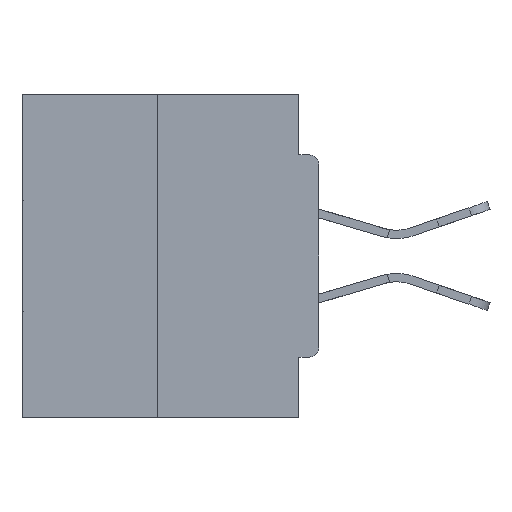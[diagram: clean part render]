
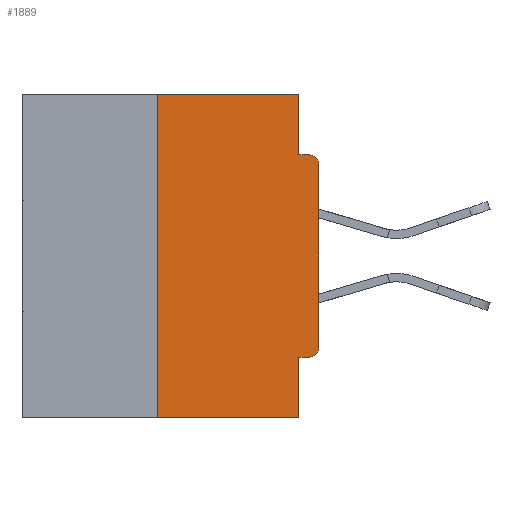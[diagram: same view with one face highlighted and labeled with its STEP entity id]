
A CAD part, left-side view. The second image highlights one B-rep face of the part: STEP entity #1889.
In plain terms, the highlighted planar face has unit normal (-1, 0, 0).
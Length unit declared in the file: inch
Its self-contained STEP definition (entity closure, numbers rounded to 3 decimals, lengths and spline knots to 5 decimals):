
#414 = CARTESIAN_POINT ( 'NONE',  ( 0., 0.015, -0.1085 ) ) ;
#616 = CARTESIAN_POINT ( 'NONE',  ( 0., 0., 0. ) ) ;
#1851 = VERTEX_POINT ( 'NONE', #23936 ) ;
#1889 = ADVANCED_FACE ( 'NONE', ( #33391 ), #14677, .F. ) ;
#1933 = CARTESIAN_POINT ( 'NONE',  ( 0., 0., -0.3915 ) ) ;
#2333 = CARTESIAN_POINT ( 'NONE',  ( 0., 0.031, -0.5 ) ) ;
#2813 = DIRECTION ( 'NONE',  ( 0., 0., -1. ) ) ;
#3236 = VERTEX_POINT ( 'NONE', #37867 ) ;
#3398 = CARTESIAN_POINT ( 'NONE',  ( 0., 0.46, 0. ) ) ;
#3588 = LINE ( 'NONE', #31933, #18099 ) ;
#3792 = ORIENTED_EDGE ( 'NONE', *, *, #18454, .T. ) ;
#4097 = LINE ( 'NONE', #2333, #38803 ) ;
#4149 = VECTOR ( 'NONE', #16017, 39.37008 ) ;
#4234 = CARTESIAN_POINT ( 'NONE',  ( 0., 0.25, 0. ) ) ;
#4863 = CIRCLE ( 'NONE', #15025, 0.015 ) ;
#6253 = EDGE_CURVE ( 'NONE', #17289, #33666, #4863, .T. ) ;
#6264 = CARTESIAN_POINT ( 'NONE',  ( 0., 0.031, -0.4065 ) ) ;
#6300 = EDGE_CURVE ( 'NONE', #36406, #16649, #18900, .T. ) ;
#7077 = LINE ( 'NONE', #13776, #25362 ) ;
#7102 = VERTEX_POINT ( 'NONE', #4234 ) ;
#8752 = LINE ( 'NONE', #3398, #20452 ) ;
#8957 = ORIENTED_EDGE ( 'NONE', *, *, #9992, .F. ) ;
#9554 = DIRECTION ( 'NONE',  ( 0., -1., 0. ) ) ;
#9948 = CARTESIAN_POINT ( 'NONE',  ( 0., 0.46, -0.5 ) ) ;
#9992 = EDGE_CURVE ( 'NONE', #15905, #16649, #4097, .T. ) ;
#11257 = CARTESIAN_POINT ( 'NONE',  ( 0., 0., -0.4065 ) ) ;
#11322 = ORIENTED_EDGE ( 'NONE', *, *, #6253, .T. ) ;
#12036 = ORIENTED_EDGE ( 'NONE', *, *, #21004, .T. ) ;
#12429 = DIRECTION ( 'NONE',  ( 0., 0., -1. ) ) ;
#12556 = VERTEX_POINT ( 'NONE', #1933 ) ;
#13629 = CARTESIAN_POINT ( 'NONE',  ( 0., 0.015, -0.3915 ) ) ;
#13650 = DIRECTION ( 'NONE',  ( 0., -1., 0. ) ) ;
#13776 = CARTESIAN_POINT ( 'NONE',  ( 0., 0.031, 0. ) ) ;
#14562 = CARTESIAN_POINT ( 'NONE',  ( 0., 0.46, 0. ) ) ;
#14677 = PLANE ( 'NONE',  #19209 ) ;
#15025 = AXIS2_PLACEMENT_3D ( 'NONE', #414, #27140, #12429 ) ;
#15644 = CARTESIAN_POINT ( 'NONE',  ( 0., 0.25, -0.5 ) ) ;
#15905 = VERTEX_POINT ( 'NONE', #6264 ) ;
#16017 = DIRECTION ( 'NONE',  ( 0., 0., 1. ) ) ;
#16440 = DIRECTION ( 'NONE',  ( 0., -1., 0. ) ) ;
#16649 = VERTEX_POINT ( 'NONE', #18668 ) ;
#16865 = EDGE_CURVE ( 'NONE', #7102, #1851, #8752, .T. ) ;
#17289 = VERTEX_POINT ( 'NONE', #26274 ) ;
#17665 = DIRECTION ( 'NONE',  ( 1., 0., 0. ) ) ;
#18099 = VECTOR ( 'NONE', #13650, 39.37008 ) ;
#18454 = EDGE_CURVE ( 'NONE', #12556, #17289, #22834, .T. ) ;
#18668 = CARTESIAN_POINT ( 'NONE',  ( 0., 0.031, -0.5 ) ) ;
#18751 = ORIENTED_EDGE ( 'NONE', *, *, #19911, .F. ) ;
#18900 = LINE ( 'NONE', #9948, #36780 ) ;
#19209 = AXIS2_PLACEMENT_3D ( 'NONE', #14562, #17665, #2813 ) ;
#19405 = CIRCLE ( 'NONE', #30527, 0.015 ) ;
#19911 = EDGE_CURVE ( 'NONE', #3236, #33666, #3588, .T. ) ;
#20408 = DIRECTION ( 'NONE',  ( 0., 1., 0. ) ) ;
#20452 = VECTOR ( 'NONE', #16440, 39.37008 ) ;
#20909 = CARTESIAN_POINT ( 'NONE',  ( 0., 0.015, -0.0935 ) ) ;
#21004 = EDGE_CURVE ( 'NONE', #21898, #12556, #19405, .T. ) ;
#21898 = VERTEX_POINT ( 'NONE', #29413 ) ;
#22062 = VECTOR ( 'NONE', #26293, 39.37008 ) ;
#22806 = ORIENTED_EDGE ( 'NONE', *, *, #16865, .F. ) ;
#22834 = LINE ( 'NONE', #616, #4149 ) ;
#23447 = LINE ( 'NONE', #26681, #22062 ) ;
#23936 = CARTESIAN_POINT ( 'NONE',  ( 0., 0.031, 0. ) ) ;
#25362 = VECTOR ( 'NONE', #29177, 39.37008 ) ;
#25604 = ORIENTED_EDGE ( 'NONE', *, *, #6300, .T. ) ;
#26274 = CARTESIAN_POINT ( 'NONE',  ( 0., 0., -0.1085 ) ) ;
#26293 = DIRECTION ( 'NONE',  ( 0., 0., 1. ) ) ;
#26408 = ORIENTED_EDGE ( 'NONE', *, *, #27761, .F. ) ;
#26681 = CARTESIAN_POINT ( 'NONE',  ( 0., 0.25, 0. ) ) ;
#27140 = DIRECTION ( 'NONE',  ( -1., 0., 0. ) ) ;
#27146 = ORIENTED_EDGE ( 'NONE', *, *, #36814, .F. ) ;
#27761 = EDGE_CURVE ( 'NONE', #1851, #3236, #7077, .T. ) ;
#29177 = DIRECTION ( 'NONE',  ( 0., 0., -1. ) ) ;
#29413 = CARTESIAN_POINT ( 'NONE',  ( 0., 0.015, -0.4065 ) ) ;
#30527 = AXIS2_PLACEMENT_3D ( 'NONE', #13629, #34251, #37660 ) ;
#31933 = CARTESIAN_POINT ( 'NONE',  ( 0., 0., -0.0935 ) ) ;
#33218 = DIRECTION ( 'NONE',  ( 0., 0., -1. ) ) ;
#33391 = FACE_OUTER_BOUND ( 'NONE', #36867, .T. ) ;
#33666 = VERTEX_POINT ( 'NONE', #20909 ) ;
#34251 = DIRECTION ( 'NONE',  ( -1., 0., 0. ) ) ;
#34562 = ORIENTED_EDGE ( 'NONE', *, *, #36161, .F. ) ;
#34742 = LINE ( 'NONE', #11257, #36601 ) ;
#36161 = EDGE_CURVE ( 'NONE', #36406, #7102, #23447, .T. ) ;
#36406 = VERTEX_POINT ( 'NONE', #15644 ) ;
#36601 = VECTOR ( 'NONE', #20408, 39.37008 ) ;
#36780 = VECTOR ( 'NONE', #9554, 39.37008 ) ;
#36814 = EDGE_CURVE ( 'NONE', #21898, #15905, #34742, .T. ) ;
#36867 = EDGE_LOOP ( 'NONE', ( #22806, #34562, #25604, #8957, #27146, #12036, #3792, #11322, #18751, #26408 ) ) ;
#37660 = DIRECTION ( 'NONE',  ( 0., 0., -1. ) ) ;
#37867 = CARTESIAN_POINT ( 'NONE',  ( 0., 0.031, -0.0935 ) ) ;
#38803 = VECTOR ( 'NONE', #33218, 39.37008 ) ;
